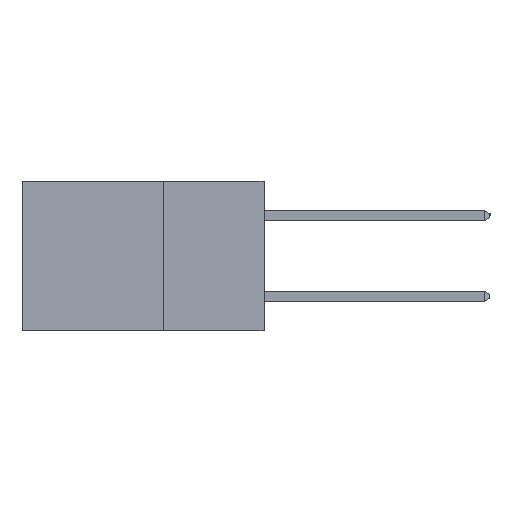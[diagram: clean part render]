
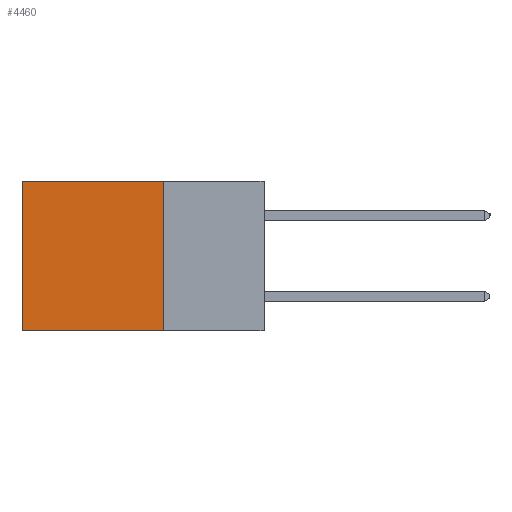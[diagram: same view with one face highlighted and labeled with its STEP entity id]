
A CAD part, left-side view. The second image highlights one B-rep face of the part: STEP entity #4460.
In plain terms, the highlighted planar face has unit normal (-1, 0, 0).
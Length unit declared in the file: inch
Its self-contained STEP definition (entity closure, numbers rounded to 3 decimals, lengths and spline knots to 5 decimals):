
#431 = DIRECTION ( 'NONE',  ( 1., 0., 0. ) ) ;
#1165 = EDGE_CURVE ( 'NONE', #6917, #1477, #2993, .T. ) ;
#1475 = VECTOR ( 'NONE', #15163, 39.37008 ) ;
#1477 = VERTEX_POINT ( 'NONE', #7899 ) ;
#1707 = EDGE_LOOP ( 'NONE', ( #10119, #15565, #11049, #14229 ) ) ;
#1916 = DIRECTION ( 'NONE',  ( 0., 0., -1. ) ) ;
#2082 = EDGE_CURVE ( 'NONE', #1477, #8137, #11502, .T. ) ;
#2822 = CARTESIAN_POINT ( 'NONE',  ( 0.2615, 0.25, -0.37 ) ) ;
#2993 = LINE ( 'NONE', #2822, #1475 ) ;
#3554 = VERTEX_POINT ( 'NONE', #4584 ) ;
#4460 = ADVANCED_FACE ( 'NONE', ( #16443 ), #15136, .F. ) ;
#4584 = CARTESIAN_POINT ( 'NONE',  ( 0.2615, 0.6, 0. ) ) ;
#4823 = DIRECTION ( 'NONE',  ( 0., 1., 0. ) ) ;
#5299 = EDGE_CURVE ( 'NONE', #3554, #8137, #13891, .T. ) ;
#5927 = CARTESIAN_POINT ( 'NONE',  ( 0.2615, 0.6, -0.37 ) ) ;
#6917 = VERTEX_POINT ( 'NONE', #8019 ) ;
#7088 = CARTESIAN_POINT ( 'NONE',  ( 0.2615, 0.25, -0.37 ) ) ;
#7228 = LINE ( 'NONE', #16324, #12428 ) ;
#7899 = CARTESIAN_POINT ( 'NONE',  ( 0.2615, 0.25, -0.37 ) ) ;
#8019 = CARTESIAN_POINT ( 'NONE',  ( 0.2615, 0.25, 0. ) ) ;
#8137 = VERTEX_POINT ( 'NONE', #5927 ) ;
#8194 = DIRECTION ( 'NONE',  ( 0., 0., -1. ) ) ;
#10119 = ORIENTED_EDGE ( 'NONE', *, *, #5299, .T. ) ;
#10465 = VECTOR ( 'NONE', #8194, 39.37008 ) ;
#11049 = ORIENTED_EDGE ( 'NONE', *, *, #1165, .F. ) ;
#11493 = EDGE_CURVE ( 'NONE', #6917, #3554, #7228, .T. ) ;
#11502 = LINE ( 'NONE', #16813, #14507 ) ;
#12428 = VECTOR ( 'NONE', #15102, 39.37008 ) ;
#13711 = CARTESIAN_POINT ( 'NONE',  ( 0.2615, 0.6, -0.37 ) ) ;
#13891 = LINE ( 'NONE', #13711, #10465 ) ;
#14229 = ORIENTED_EDGE ( 'NONE', *, *, #11493, .T. ) ;
#14507 = VECTOR ( 'NONE', #4823, 39.37008 ) ;
#15102 = DIRECTION ( 'NONE',  ( 0., 1., 0. ) ) ;
#15136 = PLANE ( 'NONE',  #16850 ) ;
#15163 = DIRECTION ( 'NONE',  ( 0., 0., -1. ) ) ;
#15565 = ORIENTED_EDGE ( 'NONE', *, *, #2082, .F. ) ;
#16324 = CARTESIAN_POINT ( 'NONE',  ( 0.2615, 0.25, 0. ) ) ;
#16443 = FACE_OUTER_BOUND ( 'NONE', #1707, .T. ) ;
#16813 = CARTESIAN_POINT ( 'NONE',  ( 0.2615, 0.25, -0.37 ) ) ;
#16850 = AXIS2_PLACEMENT_3D ( 'NONE', #7088, #431, #1916 ) ;
